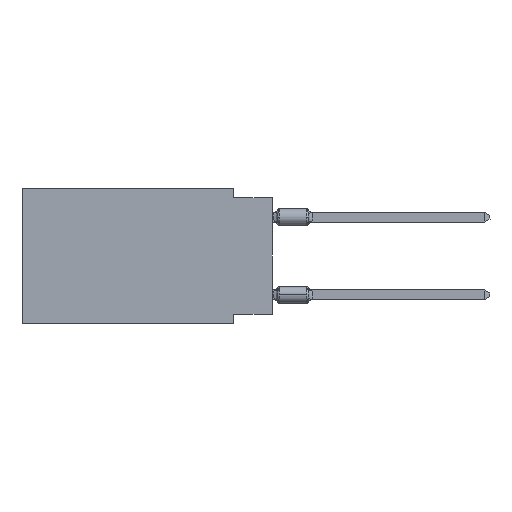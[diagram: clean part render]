
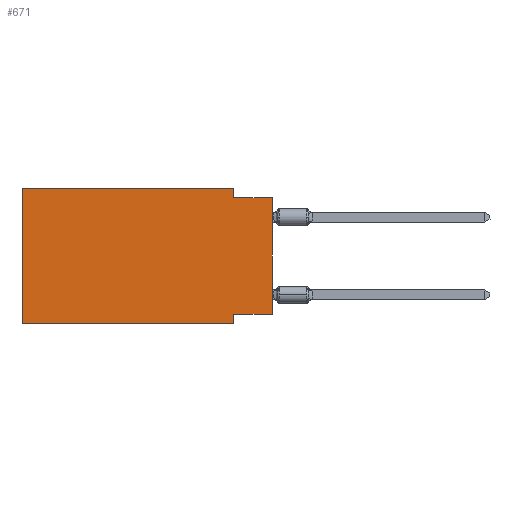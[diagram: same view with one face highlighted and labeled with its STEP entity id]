
A CAD part, left-side view. The second image highlights one B-rep face of the part: STEP entity #671.
In plain terms, the highlighted planar face has unit normal (-1, 0, 0).
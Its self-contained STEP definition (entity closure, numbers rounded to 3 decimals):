
#324 = LINE ( 'NONE', #5753, #12247 ) ;
#671 = ADVANCED_FACE ( 'NONE', ( #16755 ), #24550, .F. ) ;
#753 = VERTEX_POINT ( 'NONE', #10388 ) ;
#1278 = DIRECTION ( 'NONE',  ( 1., 0., 0. ) ) ;
#1965 = EDGE_CURVE ( 'NONE', #8914, #27505, #23504, .T. ) ;
#2754 = CARTESIAN_POINT ( 'NONE',  ( 0., 2.54, -8.89 ) ) ;
#5445 = DIRECTION ( 'NONE',  ( 0., 0., 1. ) ) ;
#5518 = DIRECTION ( 'NONE',  ( 0., 0., 1. ) ) ;
#5753 = CARTESIAN_POINT ( 'NONE',  ( 0., 16.383, 0. ) ) ;
#6177 = ORIENTED_EDGE ( 'NONE', *, *, #26235, .F. ) ;
#6622 = VERTEX_POINT ( 'NONE', #15942 ) ;
#7324 = VECTOR ( 'NONE', #16707, 1000. ) ;
#8340 = VERTEX_POINT ( 'NONE', #16322 ) ;
#8524 = VECTOR ( 'NONE', #8738, 1000. ) ;
#8738 = DIRECTION ( 'NONE',  ( 0., 0., -1. ) ) ;
#8914 = VERTEX_POINT ( 'NONE', #20764 ) ;
#9075 = CARTESIAN_POINT ( 'NONE',  ( 0., 16.383, 0. ) ) ;
#10077 = VECTOR ( 'NONE', #13367, 1000. ) ;
#10095 = CARTESIAN_POINT ( 'NONE',  ( 0., 0., -0.635 ) ) ;
#10388 = CARTESIAN_POINT ( 'NONE',  ( 0., 2.54, 0. ) ) ;
#10492 = EDGE_CURVE ( 'NONE', #32615, #8914, #33327, .T. ) ;
#11956 = VECTOR ( 'NONE', #23461, 1000. ) ;
#12247 = VECTOR ( 'NONE', #5445, 1000. ) ;
#13140 = LINE ( 'NONE', #23162, #7324 ) ;
#13306 = LINE ( 'NONE', #13494, #18983 ) ;
#13367 = DIRECTION ( 'NONE',  ( 0., -1., 0. ) ) ;
#13494 = CARTESIAN_POINT ( 'NONE',  ( 0., 0., 0. ) ) ;
#13765 = EDGE_CURVE ( 'NONE', #6622, #27505, #23416, .T. ) ;
#15419 = CARTESIAN_POINT ( 'NONE',  ( 0., 16.383, -8.89 ) ) ;
#15853 = CARTESIAN_POINT ( 'NONE',  ( 0., 16.383, 0. ) ) ;
#15942 = CARTESIAN_POINT ( 'NONE',  ( 0., 16.383, -8.89 ) ) ;
#16269 = EDGE_CURVE ( 'NONE', #24940, #8340, #28124, .T. ) ;
#16322 = CARTESIAN_POINT ( 'NONE',  ( 0., 0., -0.635 ) ) ;
#16581 = EDGE_LOOP ( 'NONE', ( #27078, #31073, #19091, #6177, #26738, #25975, #20388, #26138 ) ) ;
#16707 = DIRECTION ( 'NONE',  ( 0., -1., 0. ) ) ;
#16755 = FACE_OUTER_BOUND ( 'NONE', #16581, .T. ) ;
#16917 = VECTOR ( 'NONE', #28798, 1000. ) ;
#18188 = CARTESIAN_POINT ( 'NONE',  ( 0., 0., -8.255 ) ) ;
#18983 = VECTOR ( 'NONE', #5518, 1000. ) ;
#19091 = ORIENTED_EDGE ( 'NONE', *, *, #28419, .F. ) ;
#19443 = LINE ( 'NONE', #24038, #8524 ) ;
#19558 = EDGE_CURVE ( 'NONE', #32615, #8340, #13306, .T. ) ;
#20388 = ORIENTED_EDGE ( 'NONE', *, *, #1965, .F. ) ;
#20427 = EDGE_CURVE ( 'NONE', #6622, #27113, #324, .T. ) ;
#20764 = CARTESIAN_POINT ( 'NONE',  ( 0., 2.54, -8.255 ) ) ;
#23001 = CARTESIAN_POINT ( 'NONE',  ( 0., 2.54, -8.89 ) ) ;
#23162 = CARTESIAN_POINT ( 'NONE',  ( 0., 16.383, 0. ) ) ;
#23416 = LINE ( 'NONE', #15419, #10077 ) ;
#23461 = DIRECTION ( 'NONE',  ( 0., 1., 0. ) ) ;
#23504 = LINE ( 'NONE', #23001, #16917 ) ;
#24038 = CARTESIAN_POINT ( 'NONE',  ( 0., 2.54, 0. ) ) ;
#24395 = VECTOR ( 'NONE', #28288, 1000. ) ;
#24550 = PLANE ( 'NONE',  #28781 ) ;
#24940 = VERTEX_POINT ( 'NONE', #28600 ) ;
#25602 = CARTESIAN_POINT ( 'NONE',  ( 0., 0., -8.255 ) ) ;
#25975 = ORIENTED_EDGE ( 'NONE', *, *, #13765, .T. ) ;
#26138 = ORIENTED_EDGE ( 'NONE', *, *, #10492, .F. ) ;
#26235 = EDGE_CURVE ( 'NONE', #27113, #753, #13140, .T. ) ;
#26738 = ORIENTED_EDGE ( 'NONE', *, *, #20427, .F. ) ;
#27078 = ORIENTED_EDGE ( 'NONE', *, *, #19558, .T. ) ;
#27113 = VERTEX_POINT ( 'NONE', #15853 ) ;
#27263 = DIRECTION ( 'NONE',  ( 0., 0., -1. ) ) ;
#27505 = VERTEX_POINT ( 'NONE', #2754 ) ;
#28124 = LINE ( 'NONE', #10095, #24395 ) ;
#28288 = DIRECTION ( 'NONE',  ( 0., -1., 0. ) ) ;
#28419 = EDGE_CURVE ( 'NONE', #753, #24940, #19443, .T. ) ;
#28600 = CARTESIAN_POINT ( 'NONE',  ( 0., 2.54, -0.635 ) ) ;
#28781 = AXIS2_PLACEMENT_3D ( 'NONE', #9075, #1278, #27263 ) ;
#28798 = DIRECTION ( 'NONE',  ( 0., 0., -1. ) ) ;
#31073 = ORIENTED_EDGE ( 'NONE', *, *, #16269, .F. ) ;
#32615 = VERTEX_POINT ( 'NONE', #25602 ) ;
#33327 = LINE ( 'NONE', #18188, #11956 ) ;
